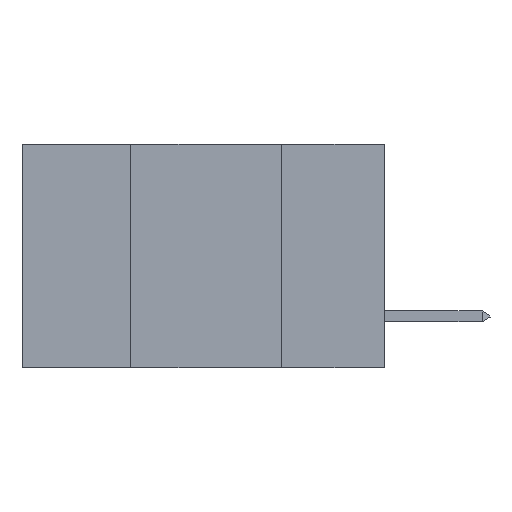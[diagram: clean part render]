
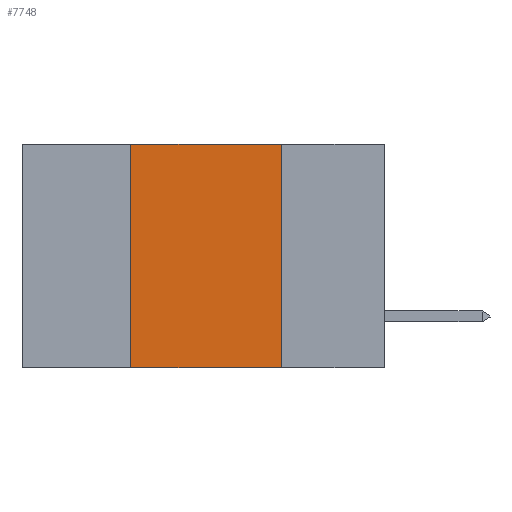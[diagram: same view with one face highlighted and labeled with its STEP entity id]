
A CAD part, left-side view. The second image highlights one B-rep face of the part: STEP entity #7748.
In plain terms, the highlighted planar face has unit normal (-1, 0, 0).
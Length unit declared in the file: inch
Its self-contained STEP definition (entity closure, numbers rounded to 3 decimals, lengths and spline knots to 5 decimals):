
#103 = VECTOR ( 'NONE', #14351, 39.37008 ) ;
#322 = LINE ( 'NONE', #15671, #103 ) ;
#685 = DIRECTION ( 'NONE',  ( 0., -1., 0. ) ) ;
#951 = LINE ( 'NONE', #15007, #9396 ) ;
#1251 = DIRECTION ( 'NONE',  ( 1., 0., 0. ) ) ;
#1446 = AXIS2_PLACEMENT_3D ( 'NONE', #5163, #1251, #15583 ) ;
#2892 = CARTESIAN_POINT ( 'NONE',  ( 0., 0.17, 0. ) ) ;
#5163 = CARTESIAN_POINT ( 'NONE',  ( 0., 0.6, 0. ) ) ;
#5342 = DIRECTION ( 'NONE',  ( 0., 0., 1. ) ) ;
#5630 = CARTESIAN_POINT ( 'NONE',  ( 0., 0.42, 0. ) ) ;
#5861 = DIRECTION ( 'NONE',  ( 0., 0., -1. ) ) ;
#6812 = CARTESIAN_POINT ( 'NONE',  ( 0., 0.42, -0.37 ) ) ;
#7190 = CARTESIAN_POINT ( 'NONE',  ( 0., 0.6, 0. ) ) ;
#7563 = FACE_OUTER_BOUND ( 'NONE', #16983, .T. ) ;
#7748 = ADVANCED_FACE ( 'NONE', ( #7563 ), #10527, .F. ) ;
#8000 = VECTOR ( 'NONE', #685, 39.37008 ) ;
#8525 = VERTEX_POINT ( 'NONE', #16353 ) ;
#9110 = CARTESIAN_POINT ( 'NONE',  ( 0., 0.42, 0. ) ) ;
#9396 = VECTOR ( 'NONE', #5861, 39.37008 ) ;
#9930 = LINE ( 'NONE', #9110, #16882 ) ;
#10028 = VERTEX_POINT ( 'NONE', #2892 ) ;
#10527 = PLANE ( 'NONE',  #1446 ) ;
#10547 = EDGE_CURVE ( 'NONE', #14445, #13468, #9930, .T. ) ;
#10653 = ORIENTED_EDGE ( 'NONE', *, *, #10547, .F. ) ;
#12312 = EDGE_CURVE ( 'NONE', #13468, #10028, #14381, .T. ) ;
#13066 = ORIENTED_EDGE ( 'NONE', *, *, #16103, .T. ) ;
#13468 = VERTEX_POINT ( 'NONE', #5630 ) ;
#14351 = DIRECTION ( 'NONE',  ( 0., -1., 0. ) ) ;
#14381 = LINE ( 'NONE', #7190, #8000 ) ;
#14445 = VERTEX_POINT ( 'NONE', #6812 ) ;
#15007 = CARTESIAN_POINT ( 'NONE',  ( 0., 0.17, 0. ) ) ;
#15583 = DIRECTION ( 'NONE',  ( 0., 0., -1. ) ) ;
#15643 = ORIENTED_EDGE ( 'NONE', *, *, #15824, .F. ) ;
#15671 = CARTESIAN_POINT ( 'NONE',  ( 0., 0.6, -0.37 ) ) ;
#15824 = EDGE_CURVE ( 'NONE', #10028, #8525, #951, .T. ) ;
#16103 = EDGE_CURVE ( 'NONE', #14445, #8525, #322, .T. ) ;
#16353 = CARTESIAN_POINT ( 'NONE',  ( 0., 0.17, -0.37 ) ) ;
#16412 = ORIENTED_EDGE ( 'NONE', *, *, #12312, .F. ) ;
#16882 = VECTOR ( 'NONE', #5342, 39.37008 ) ;
#16983 = EDGE_LOOP ( 'NONE', ( #15643, #16412, #10653, #13066 ) ) ;
